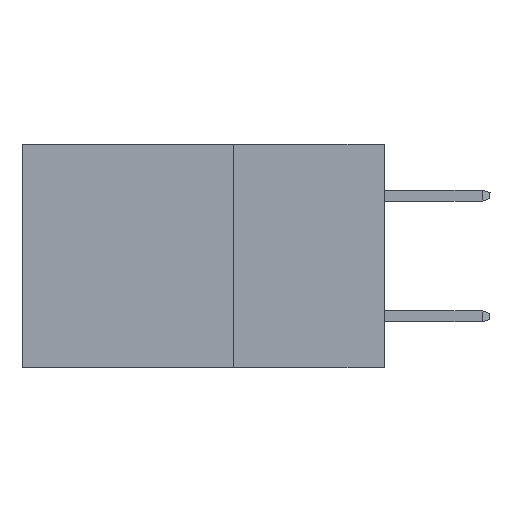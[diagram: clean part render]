
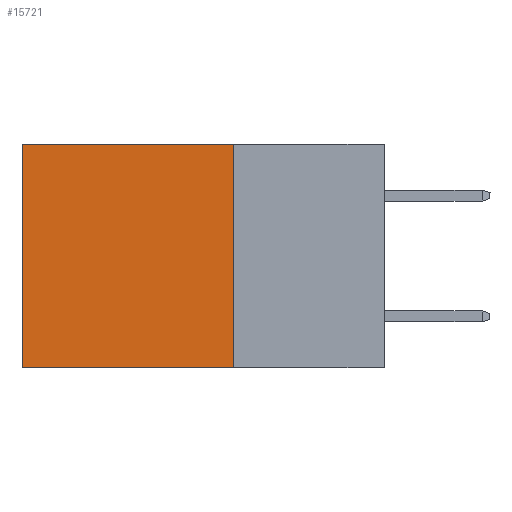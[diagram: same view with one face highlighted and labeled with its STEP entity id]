
A CAD part, left-side view. The second image highlights one B-rep face of the part: STEP entity #15721.
In plain terms, the highlighted planar face has unit normal (-1, 0, 0).
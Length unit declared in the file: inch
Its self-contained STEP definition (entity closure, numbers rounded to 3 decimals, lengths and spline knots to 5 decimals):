
#44 = DIRECTION ( 'NONE',  ( 0., 0., -1. ) ) ;
#466 = EDGE_CURVE ( 'NONE', #9067, #10794, #12235, .T. ) ;
#926 = CARTESIAN_POINT ( 'NONE',  ( 0.298, 0.25, -0.37 ) ) ;
#2210 = ORIENTED_EDGE ( 'NONE', *, *, #13447, .F. ) ;
#2232 = EDGE_CURVE ( 'NONE', #2676, #10794, #16185, .T. ) ;
#2303 = VERTEX_POINT ( 'NONE', #3093 ) ;
#2676 = VERTEX_POINT ( 'NONE', #926 ) ;
#3093 = CARTESIAN_POINT ( 'NONE',  ( 0.298, 0.25, 0. ) ) ;
#3190 = AXIS2_PLACEMENT_3D ( 'NONE', #7240, #8684, #44 ) ;
#3524 = EDGE_LOOP ( 'NONE', ( #17367, #4095, #2210, #17405 ) ) ;
#4095 = ORIENTED_EDGE ( 'NONE', *, *, #2232, .F. ) ;
#5170 = VECTOR ( 'NONE', #15767, 39.37008 ) ;
#5197 = DIRECTION ( 'NONE',  ( 0., 0., -1. ) ) ;
#5404 = CARTESIAN_POINT ( 'NONE',  ( 0.298, 0.25, -0.37 ) ) ;
#5589 = LINE ( 'NONE', #6909, #12347 ) ;
#5647 = DIRECTION ( 'NONE',  ( 0., 1., 0. ) ) ;
#5741 = CARTESIAN_POINT ( 'NONE',  ( 0.298, 0.25, 0. ) ) ;
#6674 = FACE_OUTER_BOUND ( 'NONE', #3524, .T. ) ;
#6909 = CARTESIAN_POINT ( 'NONE',  ( 0.298, 0.25, 0. ) ) ;
#7240 = CARTESIAN_POINT ( 'NONE',  ( 0.298, 0.25, 0. ) ) ;
#8136 = LINE ( 'NONE', #5741, #5170 ) ;
#8378 = DIRECTION ( 'NONE',  ( 0., 0., -1. ) ) ;
#8459 = VECTOR ( 'NONE', #5197, 39.37008 ) ;
#8684 = DIRECTION ( 'NONE',  ( 1., 0., 0. ) ) ;
#9067 = VERTEX_POINT ( 'NONE', #12879 ) ;
#9071 = EDGE_CURVE ( 'NONE', #2303, #9067, #8136, .T. ) ;
#9957 = CARTESIAN_POINT ( 'NONE',  ( 0.298, 0.6, 0. ) ) ;
#10721 = CARTESIAN_POINT ( 'NONE',  ( 0.298, 0.6, -0.37 ) ) ;
#10794 = VERTEX_POINT ( 'NONE', #10721 ) ;
#12235 = LINE ( 'NONE', #9957, #8459 ) ;
#12347 = VECTOR ( 'NONE', #8378, 39.37008 ) ;
#12879 = CARTESIAN_POINT ( 'NONE',  ( 0.298, 0.6, 0. ) ) ;
#13447 = EDGE_CURVE ( 'NONE', #2303, #2676, #5589, .T. ) ;
#15721 = ADVANCED_FACE ( 'NONE', ( #6674 ), #15777, .F. ) ;
#15767 = DIRECTION ( 'NONE',  ( 0., 1., 0. ) ) ;
#15777 = PLANE ( 'NONE',  #3190 ) ;
#16185 = LINE ( 'NONE', #5404, #16631 ) ;
#16631 = VECTOR ( 'NONE', #5647, 39.37008 ) ;
#17367 = ORIENTED_EDGE ( 'NONE', *, *, #466, .T. ) ;
#17405 = ORIENTED_EDGE ( 'NONE', *, *, #9071, .T. ) ;
